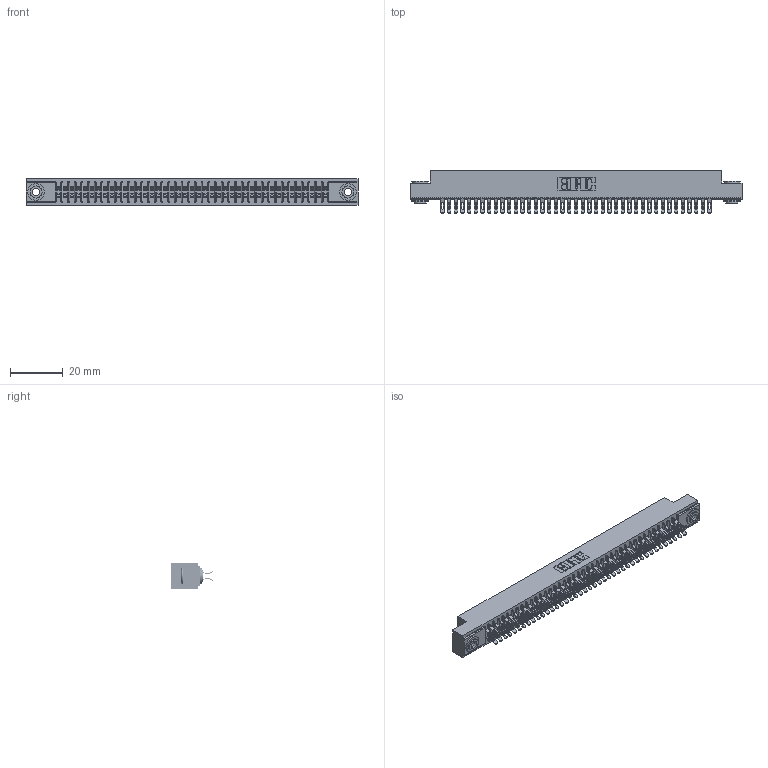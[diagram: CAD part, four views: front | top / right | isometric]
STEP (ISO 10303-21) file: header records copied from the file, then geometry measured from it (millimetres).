
FILE_DESCRIPTION (( 'STEP AP203' ), '1' );
FILE_NAME ('341-082-555-203.STEP', '2018-08-07T22:16:28', ( '' ), ( '' ), 'SwSTEP 2.0', 'SolidWorks 2016', '' );
FILE_SCHEMA (( 'CONFIG_CONTROL_DESIGN' ));
Length unit declared in the file: inch
Products named in the file (4): 341-082-555-203; 341 Part_.156 (3.96) Dia Mounting Holes; 341-292-001_341-292-155; 345-250-002_345-250-002-102
Assembly tree (85 placements, depth 2):
  341-082-555-203
    341 Part_.156 (3.96) Dia Mounting Holes
    341-292-001_341-292-155  x82
    345-250-002_345-250-002-102  x2
Bounding box: 126.36 x 16.31 x 10.16 mm (x, y, z)
Volume: 9436.1 mm3; surface area: 17632.1 mm2
Topology: 85 solids, 85 shells, 6564 faces, 19575 edges, 12742 vertices
Faces by surface type: plane 3536, cylinder 2856, sphere 84, torus 80, cone 8
Entity records: 51287 total; most frequent: CARTESIAN_POINT 8522, ORIENTED_EDGE 8450, DIRECTION 8277, EDGE_CURVE 4225, LINE 3387, VECTOR 3387, VERTEX_POINT 2674, AXIS2_PLACEMENT_3D 2445
